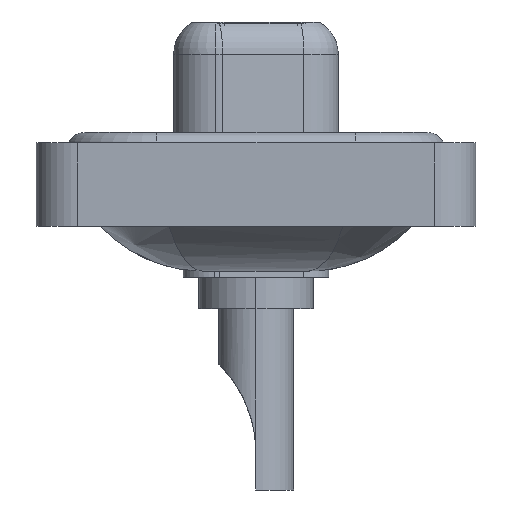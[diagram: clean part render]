
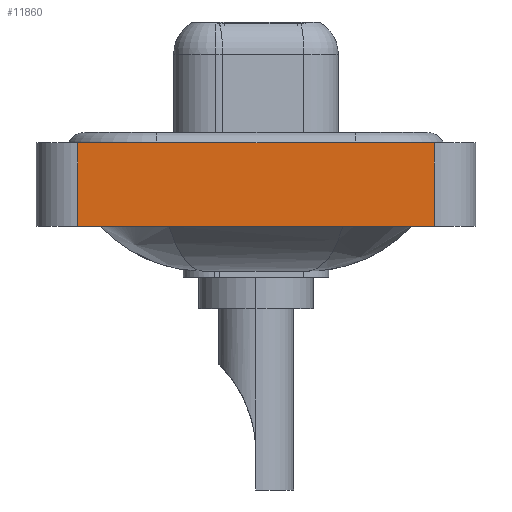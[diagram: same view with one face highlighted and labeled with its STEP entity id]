
A CAD part, left-side view. The second image highlights one B-rep face of the part: STEP entity #11860.
In plain terms, the highlighted planar face has unit normal (-1, 0, 0).
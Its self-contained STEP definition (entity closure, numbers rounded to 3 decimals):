
#1234 = LINE ( 'NONE', #17897, #8632 ) ;
#2206 = CARTESIAN_POINT ( 'NONE',  ( -7.3, -8.55, -3.6 ) ) ;
#2241 = DIRECTION ( 'NONE',  ( 0., 0., 1. ) ) ;
#2269 = EDGE_CURVE ( 'NONE', #10556, #11536, #10523, .T. ) ;
#2435 = VECTOR ( 'NONE', #11804, 1000. ) ;
#2677 = DIRECTION ( 'NONE',  ( 0., -1., 0. ) ) ;
#2763 = DIRECTION ( 'NONE',  ( 0., 0., 1. ) ) ;
#3125 = ORIENTED_EDGE ( 'NONE', *, *, #2269, .T. ) ;
#3185 = EDGE_CURVE ( 'NONE', #11248, #6295, #1234, .T. ) ;
#3601 = PLANE ( 'NONE',  #11003 ) ;
#5354 = ORIENTED_EDGE ( 'NONE', *, *, #3185, .F. ) ;
#6295 = VERTEX_POINT ( 'NONE', #7238 ) ;
#6437 = DIRECTION ( 'NONE',  ( 0., 0., 1. ) ) ;
#6978 = VECTOR ( 'NONE', #2763, 1000. ) ;
#7238 = CARTESIAN_POINT ( 'NONE',  ( -7.3, -8.55, 0.4 ) ) ;
#7903 = CARTESIAN_POINT ( 'NONE',  ( -7.3, -8.55, -3.6 ) ) ;
#8152 = LINE ( 'NONE', #12263, #6978 ) ;
#8632 = VECTOR ( 'NONE', #2677, 1000. ) ;
#9131 = EDGE_CURVE ( 'NONE', #10556, #11248, #8152, .T. ) ;
#9627 = CARTESIAN_POINT ( 'NONE',  ( -7.3, 8.55, -3.6 ) ) ;
#10523 = LINE ( 'NONE', #2206, #2435 ) ;
#10534 = CARTESIAN_POINT ( 'NONE',  ( -7.3, -8.55, -3.6 ) ) ;
#10556 = VERTEX_POINT ( 'NONE', #9627 ) ;
#11003 = AXIS2_PLACEMENT_3D ( 'NONE', #10534, #17536, #6437 ) ;
#11248 = VERTEX_POINT ( 'NONE', #13224 ) ;
#11536 = VERTEX_POINT ( 'NONE', #7903 ) ;
#11732 = EDGE_LOOP ( 'NONE', ( #16764, #5354, #15425, #3125 ) ) ;
#11804 = DIRECTION ( 'NONE',  ( 0., -1., 0. ) ) ;
#11860 = ADVANCED_FACE ( 'NONE', ( #17456 ), #3601, .T. ) ;
#12100 = LINE ( 'NONE', #17820, #13197 ) ;
#12263 = CARTESIAN_POINT ( 'NONE',  ( -7.3, 8.55, -3.6 ) ) ;
#13197 = VECTOR ( 'NONE', #2241, 1000. ) ;
#13224 = CARTESIAN_POINT ( 'NONE',  ( -7.3, 8.55, 0.4 ) ) ;
#13521 = EDGE_CURVE ( 'NONE', #11536, #6295, #12100, .T. ) ;
#15425 = ORIENTED_EDGE ( 'NONE', *, *, #9131, .F. ) ;
#16764 = ORIENTED_EDGE ( 'NONE', *, *, #13521, .T. ) ;
#17456 = FACE_OUTER_BOUND ( 'NONE', #11732, .T. ) ;
#17536 = DIRECTION ( 'NONE',  ( -1., 0., 0. ) ) ;
#17820 = CARTESIAN_POINT ( 'NONE',  ( -7.3, -8.55, -3.6 ) ) ;
#17897 = CARTESIAN_POINT ( 'NONE',  ( -7.3, -8.55, 0.4 ) ) ;
